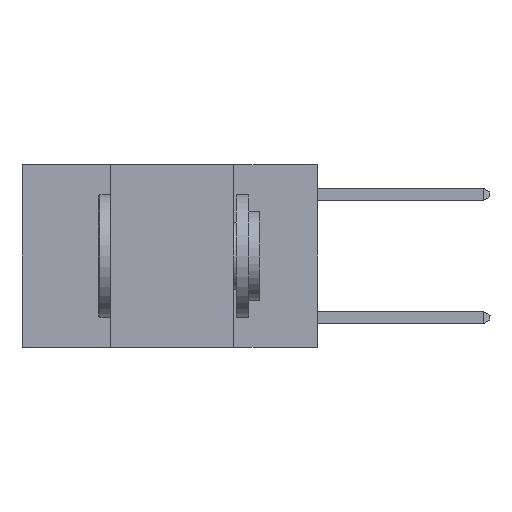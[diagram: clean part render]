
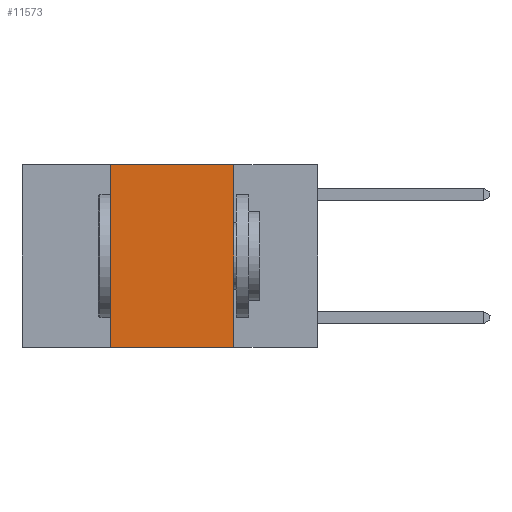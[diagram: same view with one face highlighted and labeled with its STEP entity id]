
A CAD part, left-side view. The second image highlights one B-rep face of the part: STEP entity #11573.
In plain terms, the highlighted planar face has unit normal (-1, 0, 0).
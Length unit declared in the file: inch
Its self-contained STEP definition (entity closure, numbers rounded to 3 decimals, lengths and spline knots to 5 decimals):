
#214 = ORIENTED_EDGE ( 'NONE', *, *, #9544, .F. ) ;
#604 = DIRECTION ( 'NONE',  ( 1., 0., 0. ) ) ;
#613 = VERTEX_POINT ( 'NONE', #18880 ) ;
#1273 = LINE ( 'NONE', #8326, #18849 ) ;
#1977 = VECTOR ( 'NONE', #12751, 39.37008 ) ;
#2598 = CARTESIAN_POINT ( 'NONE',  ( 0., 0.42, 0. ) ) ;
#3164 = CARTESIAN_POINT ( 'NONE',  ( 0., 0.17, -0.37 ) ) ;
#3449 = VERTEX_POINT ( 'NONE', #3814 ) ;
#3718 = LINE ( 'NONE', #5065, #14558 ) ;
#3814 = CARTESIAN_POINT ( 'NONE',  ( 0., 0.17, 0. ) ) ;
#4041 = EDGE_CURVE ( 'NONE', #4556, #613, #17475, .T. ) ;
#4556 = VERTEX_POINT ( 'NONE', #16844 ) ;
#4929 = CARTESIAN_POINT ( 'NONE',  ( 0., 0.6, 0. ) ) ;
#5065 = CARTESIAN_POINT ( 'NONE',  ( 0., 0.6, 0. ) ) ;
#5486 = DIRECTION ( 'NONE',  ( 0., -1., 0. ) ) ;
#5842 = LINE ( 'NONE', #14197, #1977 ) ;
#7660 = FACE_OUTER_BOUND ( 'NONE', #18437, .T. ) ;
#8326 = CARTESIAN_POINT ( 'NONE',  ( 0., 0.6, -0.37 ) ) ;
#8501 = VERTEX_POINT ( 'NONE', #3164 ) ;
#9389 = PLANE ( 'NONE',  #9947 ) ;
#9544 = EDGE_CURVE ( 'NONE', #3449, #8501, #5842, .T. ) ;
#9947 = AXIS2_PLACEMENT_3D ( 'NONE', #4929, #604, #10865 ) ;
#10865 = DIRECTION ( 'NONE',  ( 0., 0., -1. ) ) ;
#11109 = EDGE_CURVE ( 'NONE', #613, #3449, #3718, .T. ) ;
#11573 = ADVANCED_FACE ( 'NONE', ( #7660 ), #9389, .F. ) ;
#12441 = ORIENTED_EDGE ( 'NONE', *, *, #11109, .F. ) ;
#12751 = DIRECTION ( 'NONE',  ( 0., 0., -1. ) ) ;
#13699 = VECTOR ( 'NONE', #18633, 39.37008 ) ;
#14197 = CARTESIAN_POINT ( 'NONE',  ( 0., 0.17, 0. ) ) ;
#14558 = VECTOR ( 'NONE', #15339, 39.37008 ) ;
#15339 = DIRECTION ( 'NONE',  ( 0., -1., 0. ) ) ;
#16251 = ORIENTED_EDGE ( 'NONE', *, *, #4041, .F. ) ;
#16697 = ORIENTED_EDGE ( 'NONE', *, *, #18621, .T. ) ;
#16844 = CARTESIAN_POINT ( 'NONE',  ( 0., 0.42, -0.37 ) ) ;
#17475 = LINE ( 'NONE', #2598, #13699 ) ;
#18437 = EDGE_LOOP ( 'NONE', ( #214, #12441, #16251, #16697 ) ) ;
#18621 = EDGE_CURVE ( 'NONE', #4556, #8501, #1273, .T. ) ;
#18633 = DIRECTION ( 'NONE',  ( 0., 0., 1. ) ) ;
#18849 = VECTOR ( 'NONE', #5486, 39.37008 ) ;
#18880 = CARTESIAN_POINT ( 'NONE',  ( 0., 0.42, 0. ) ) ;
